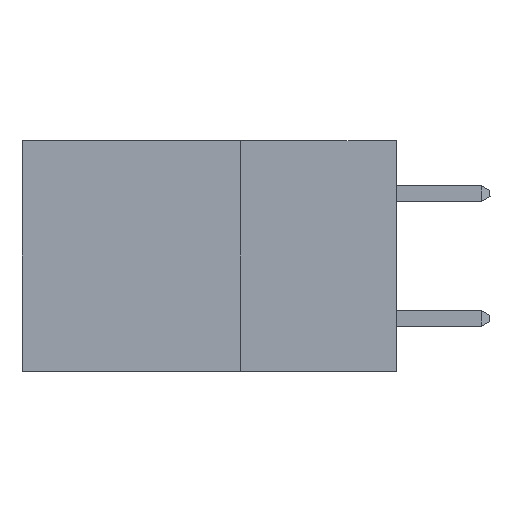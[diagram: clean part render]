
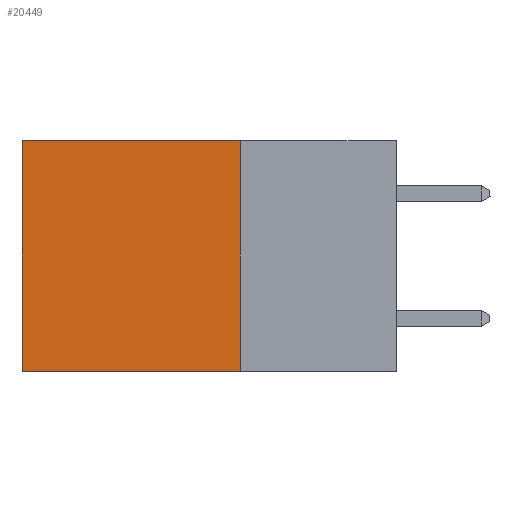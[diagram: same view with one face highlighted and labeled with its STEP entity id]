
A CAD part, left-side view. The second image highlights one B-rep face of the part: STEP entity #20449.
In plain terms, the highlighted planar face has unit normal (-1, 0, 0).
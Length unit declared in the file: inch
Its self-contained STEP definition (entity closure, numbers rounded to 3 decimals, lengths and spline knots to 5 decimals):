
#601 = VECTOR ( 'NONE', #19050, 39.37008 ) ;
#723 = LINE ( 'NONE', #15767, #8163 ) ;
#785 = DIRECTION ( 'NONE',  ( 0., 1., 0. ) ) ;
#918 = FACE_OUTER_BOUND ( 'NONE', #5372, .T. ) ;
#1487 = EDGE_CURVE ( 'NONE', #18531, #16661, #19610, .T. ) ;
#1522 = DIRECTION ( 'NONE',  ( 0., 0., -1. ) ) ;
#2123 = CARTESIAN_POINT ( 'NONE',  ( 0.298, 0.6, -0.37 ) ) ;
#2239 = PLANE ( 'NONE',  #21175 ) ;
#3027 = CARTESIAN_POINT ( 'NONE',  ( 0.298, 0.25, -0.37 ) ) ;
#5340 = CARTESIAN_POINT ( 'NONE',  ( 0.298, 0.25, -0.37 ) ) ;
#5372 = EDGE_LOOP ( 'NONE', ( #7731, #20482, #12528, #13107 ) ) ;
#6855 = EDGE_CURVE ( 'NONE', #10644, #16661, #15108, .T. ) ;
#7382 = VECTOR ( 'NONE', #785, 39.37008 ) ;
#7731 = ORIENTED_EDGE ( 'NONE', *, *, #1487, .T. ) ;
#7912 = EDGE_CURVE ( 'NONE', #18284, #10644, #723, .T. ) ;
#8163 = VECTOR ( 'NONE', #15843, 39.37008 ) ;
#10644 = VERTEX_POINT ( 'NONE', #5340 ) ;
#10781 = CARTESIAN_POINT ( 'NONE',  ( 0.298, 0.6, 0. ) ) ;
#11706 = CARTESIAN_POINT ( 'NONE',  ( 0.298, 0.25, 0. ) ) ;
#12209 = LINE ( 'NONE', #11706, #7382 ) ;
#12528 = ORIENTED_EDGE ( 'NONE', *, *, #7912, .F. ) ;
#12864 = CARTESIAN_POINT ( 'NONE',  ( 0.298, 0.6, 0. ) ) ;
#13107 = ORIENTED_EDGE ( 'NONE', *, *, #22769, .T. ) ;
#14064 = CARTESIAN_POINT ( 'NONE',  ( 0.298, 0.25, 0. ) ) ;
#14786 = VECTOR ( 'NONE', #1522, 39.37008 ) ;
#14894 = DIRECTION ( 'NONE',  ( 0., 0., -1. ) ) ;
#15042 = CARTESIAN_POINT ( 'NONE',  ( 0.298, 0.25, 0. ) ) ;
#15108 = LINE ( 'NONE', #3027, #601 ) ;
#15767 = CARTESIAN_POINT ( 'NONE',  ( 0.298, 0.25, 0. ) ) ;
#15843 = DIRECTION ( 'NONE',  ( 0., 0., -1. ) ) ;
#16661 = VERTEX_POINT ( 'NONE', #2123 ) ;
#16664 = DIRECTION ( 'NONE',  ( 1., 0., 0. ) ) ;
#18284 = VERTEX_POINT ( 'NONE', #14064 ) ;
#18531 = VERTEX_POINT ( 'NONE', #12864 ) ;
#19050 = DIRECTION ( 'NONE',  ( 0., 1., 0. ) ) ;
#19610 = LINE ( 'NONE', #10781, #14786 ) ;
#20449 = ADVANCED_FACE ( 'NONE', ( #918 ), #2239, .F. ) ;
#20482 = ORIENTED_EDGE ( 'NONE', *, *, #6855, .F. ) ;
#21175 = AXIS2_PLACEMENT_3D ( 'NONE', #15042, #16664, #14894 ) ;
#22769 = EDGE_CURVE ( 'NONE', #18284, #18531, #12209, .T. ) ;
